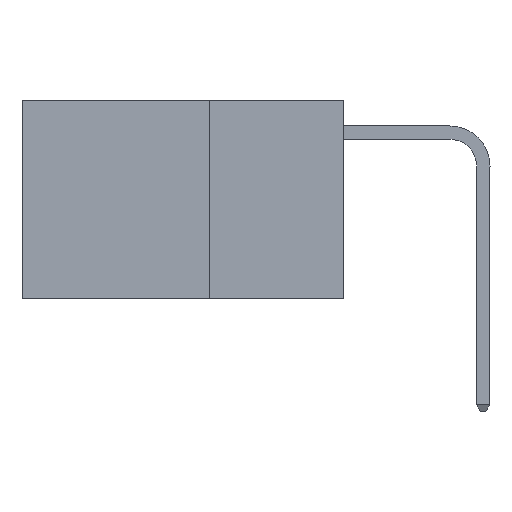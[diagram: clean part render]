
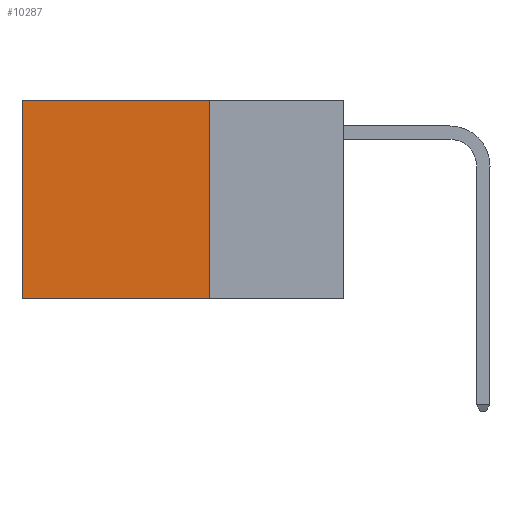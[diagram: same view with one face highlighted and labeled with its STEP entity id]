
A CAD part, left-side view. The second image highlights one B-rep face of the part: STEP entity #10287.
In plain terms, the highlighted planar face has unit normal (-1, 0, 0).
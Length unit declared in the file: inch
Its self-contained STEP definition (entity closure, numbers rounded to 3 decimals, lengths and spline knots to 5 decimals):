
#823 = CARTESIAN_POINT ( 'NONE',  ( 0.2625, 0.25, -0.37 ) ) ;
#919 = VECTOR ( 'NONE', #9876, 39.37008 ) ;
#1034 = CARTESIAN_POINT ( 'NONE',  ( 0.2625, 0.6, 0. ) ) ;
#1063 = LINE ( 'NONE', #9572, #14008 ) ;
#1214 = ORIENTED_EDGE ( 'NONE', *, *, #14052, .T. ) ;
#2904 = VERTEX_POINT ( 'NONE', #6171 ) ;
#3767 = LINE ( 'NONE', #1034, #7625 ) ;
#4599 = EDGE_CURVE ( 'NONE', #10597, #14416, #9242, .T. ) ;
#4962 = CARTESIAN_POINT ( 'NONE',  ( 0.2625, 0.25, 0. ) ) ;
#5927 = ORIENTED_EDGE ( 'NONE', *, *, #8854, .F. ) ;
#6171 = CARTESIAN_POINT ( 'NONE',  ( 0.2625, 0.6, -0.37 ) ) ;
#6630 = ORIENTED_EDGE ( 'NONE', *, *, #4599, .F. ) ;
#7625 = VECTOR ( 'NONE', #12507, 39.37008 ) ;
#8269 = DIRECTION ( 'NONE',  ( 0., 0., -1. ) ) ;
#8854 = EDGE_CURVE ( 'NONE', #14416, #2904, #11133, .T. ) ;
#9205 = VECTOR ( 'NONE', #9817, 39.37008 ) ;
#9242 = LINE ( 'NONE', #9943, #9205 ) ;
#9277 = EDGE_LOOP ( 'NONE', ( #10329, #5927, #6630, #1214 ) ) ;
#9572 = CARTESIAN_POINT ( 'NONE',  ( 0.2625, 0.25, 0. ) ) ;
#9633 = FACE_OUTER_BOUND ( 'NONE', #9277, .T. ) ;
#9817 = DIRECTION ( 'NONE',  ( 0., 0., -1. ) ) ;
#9876 = DIRECTION ( 'NONE',  ( 0., 1., 0. ) ) ;
#9943 = CARTESIAN_POINT ( 'NONE',  ( 0.2625, 0.25, 0. ) ) ;
#10287 = ADVANCED_FACE ( 'NONE', ( #9633 ), #14141, .F. ) ;
#10329 = ORIENTED_EDGE ( 'NONE', *, *, #15559, .T. ) ;
#10597 = VERTEX_POINT ( 'NONE', #4962 ) ;
#11133 = LINE ( 'NONE', #823, #919 ) ;
#11323 = CARTESIAN_POINT ( 'NONE',  ( 0.2625, 0.25, -0.37 ) ) ;
#12507 = DIRECTION ( 'NONE',  ( 0., 0., -1. ) ) ;
#13229 = DIRECTION ( 'NONE',  ( 0., 1., 0. ) ) ;
#13531 = AXIS2_PLACEMENT_3D ( 'NONE', #14182, #15277, #8269 ) ;
#14008 = VECTOR ( 'NONE', #13229, 39.37008 ) ;
#14052 = EDGE_CURVE ( 'NONE', #10597, #14099, #1063, .T. ) ;
#14099 = VERTEX_POINT ( 'NONE', #15454 ) ;
#14141 = PLANE ( 'NONE',  #13531 ) ;
#14182 = CARTESIAN_POINT ( 'NONE',  ( 0.2625, 0.25, 0. ) ) ;
#14416 = VERTEX_POINT ( 'NONE', #11323 ) ;
#15277 = DIRECTION ( 'NONE',  ( 1., 0., 0. ) ) ;
#15454 = CARTESIAN_POINT ( 'NONE',  ( 0.2625, 0.6, 0. ) ) ;
#15559 = EDGE_CURVE ( 'NONE', #14099, #2904, #3767, .T. ) ;
